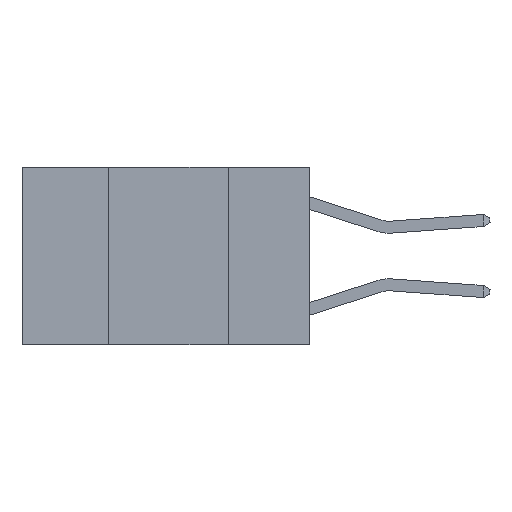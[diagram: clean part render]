
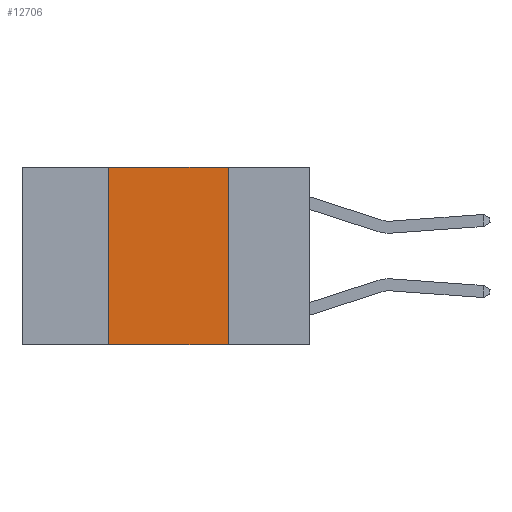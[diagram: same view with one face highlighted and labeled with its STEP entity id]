
A CAD part, left-side view. The second image highlights one B-rep face of the part: STEP entity #12706.
In plain terms, the highlighted planar face has unit normal (-1, 0, 0).
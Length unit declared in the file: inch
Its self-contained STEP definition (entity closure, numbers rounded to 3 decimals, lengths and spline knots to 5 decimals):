
#97 = CARTESIAN_POINT ( 'NONE',  ( 0., 0.6, 0. ) ) ;
#1208 = LINE ( 'NONE', #9813, #8350 ) ;
#1280 = VERTEX_POINT ( 'NONE', #10511 ) ;
#1534 = CARTESIAN_POINT ( 'NONE',  ( 0., 0.6, 0. ) ) ;
#1998 = LINE ( 'NONE', #8777, #3514 ) ;
#2524 = PLANE ( 'NONE',  #8858 ) ;
#2846 = ORIENTED_EDGE ( 'NONE', *, *, #8093, .F. ) ;
#3452 = FACE_OUTER_BOUND ( 'NONE', #6036, .T. ) ;
#3514 = VECTOR ( 'NONE', #6359, 39.37008 ) ;
#3589 = DIRECTION ( 'NONE',  ( 0., 0., -1. ) ) ;
#3888 = VERTEX_POINT ( 'NONE', #12793 ) ;
#5756 = LINE ( 'NONE', #97, #7196 ) ;
#6036 = EDGE_LOOP ( 'NONE', ( #13327, #2846, #13407, #8511 ) ) ;
#6098 = CARTESIAN_POINT ( 'NONE',  ( 0., 0.42, 0. ) ) ;
#6359 = DIRECTION ( 'NONE',  ( 0., 0., -1. ) ) ;
#6536 = EDGE_CURVE ( 'NONE', #12170, #1280, #1998, .T. ) ;
#7196 = VECTOR ( 'NONE', #8868, 39.37008 ) ;
#7673 = DIRECTION ( 'NONE',  ( 0., -1., 0. ) ) ;
#8093 = EDGE_CURVE ( 'NONE', #9152, #12170, #5756, .T. ) ;
#8350 = VECTOR ( 'NONE', #7673, 39.37008 ) ;
#8511 = ORIENTED_EDGE ( 'NONE', *, *, #8525, .T. ) ;
#8525 = EDGE_CURVE ( 'NONE', #3888, #1280, #1208, .T. ) ;
#8777 = CARTESIAN_POINT ( 'NONE',  ( 0., 0.17, 0. ) ) ;
#8858 = AXIS2_PLACEMENT_3D ( 'NONE', #1534, #12293, #3589 ) ;
#8868 = DIRECTION ( 'NONE',  ( 0., -1., 0. ) ) ;
#9152 = VERTEX_POINT ( 'NONE', #6098 ) ;
#9718 = EDGE_CURVE ( 'NONE', #3888, #9152, #10328, .T. ) ;
#9813 = CARTESIAN_POINT ( 'NONE',  ( 0., 0.6, -0.37 ) ) ;
#10328 = LINE ( 'NONE', #11474, #10602 ) ;
#10511 = CARTESIAN_POINT ( 'NONE',  ( 0., 0.17, -0.37 ) ) ;
#10540 = DIRECTION ( 'NONE',  ( 0., 0., 1. ) ) ;
#10602 = VECTOR ( 'NONE', #10540, 39.37008 ) ;
#11474 = CARTESIAN_POINT ( 'NONE',  ( 0., 0.42, 0. ) ) ;
#12170 = VERTEX_POINT ( 'NONE', #12480 ) ;
#12293 = DIRECTION ( 'NONE',  ( 1., 0., 0. ) ) ;
#12480 = CARTESIAN_POINT ( 'NONE',  ( 0., 0.17, 0. ) ) ;
#12706 = ADVANCED_FACE ( 'NONE', ( #3452 ), #2524, .F. ) ;
#12793 = CARTESIAN_POINT ( 'NONE',  ( 0., 0.42, -0.37 ) ) ;
#13327 = ORIENTED_EDGE ( 'NONE', *, *, #6536, .F. ) ;
#13407 = ORIENTED_EDGE ( 'NONE', *, *, #9718, .F. ) ;
